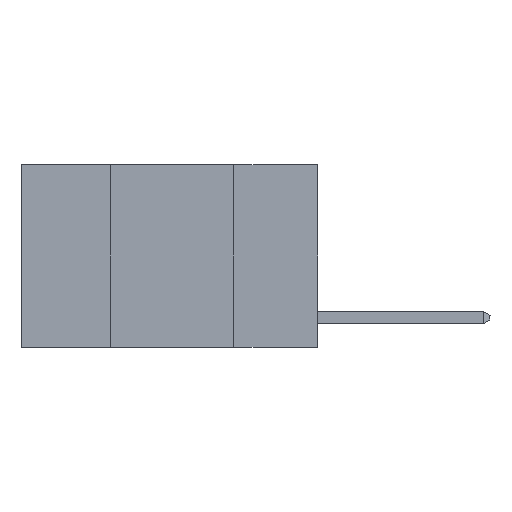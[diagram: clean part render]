
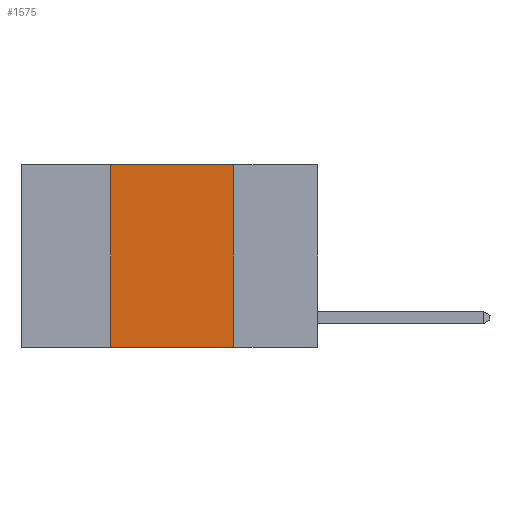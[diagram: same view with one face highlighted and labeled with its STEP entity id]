
A CAD part, left-side view. The second image highlights one B-rep face of the part: STEP entity #1575.
In plain terms, the highlighted planar face has unit normal (-1, 0, 0).
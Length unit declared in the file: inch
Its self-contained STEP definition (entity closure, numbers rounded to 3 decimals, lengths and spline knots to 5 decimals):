
#529 = VECTOR ( 'NONE', #25299, 39.37008 ) ;
#1575 = ADVANCED_FACE ( 'NONE', ( #6108 ), #21739, .F. ) ;
#1997 = LINE ( 'NONE', #19917, #529 ) ;
#3007 = VERTEX_POINT ( 'NONE', #13821 ) ;
#3085 = EDGE_CURVE ( 'NONE', #11057, #13560, #20393, .T. ) ;
#3629 = ORIENTED_EDGE ( 'NONE', *, *, #12092, .F. ) ;
#4071 = DIRECTION ( 'NONE',  ( 0., 0., -1. ) ) ;
#4110 = EDGE_LOOP ( 'NONE', ( #23858, #20177, #3629, #20662 ) ) ;
#4261 = EDGE_CURVE ( 'NONE', #12815, #3007, #12194, .T. ) ;
#6108 = FACE_OUTER_BOUND ( 'NONE', #4110, .T. ) ;
#6417 = DIRECTION ( 'NONE',  ( 0., -1., 0. ) ) ;
#6546 = CARTESIAN_POINT ( 'NONE',  ( 0., 0.6, 0. ) ) ;
#6825 = DIRECTION ( 'NONE',  ( 0., -1., 0. ) ) ;
#7036 = LINE ( 'NONE', #15425, #8098 ) ;
#8098 = VECTOR ( 'NONE', #8956, 39.37008 ) ;
#8956 = DIRECTION ( 'NONE',  ( 0., 0., 1. ) ) ;
#9853 = CARTESIAN_POINT ( 'NONE',  ( 0., 0.17, -0.37 ) ) ;
#10684 = CARTESIAN_POINT ( 'NONE',  ( 0., 0.6, -0.37 ) ) ;
#11057 = VERTEX_POINT ( 'NONE', #24647 ) ;
#11877 = CARTESIAN_POINT ( 'NONE',  ( 0., 0.6, 0. ) ) ;
#12092 = EDGE_CURVE ( 'NONE', #11057, #12815, #7036, .T. ) ;
#12194 = LINE ( 'NONE', #6546, #23670 ) ;
#12815 = VERTEX_POINT ( 'NONE', #24741 ) ;
#13560 = VERTEX_POINT ( 'NONE', #9853 ) ;
#13821 = CARTESIAN_POINT ( 'NONE',  ( 0., 0.17, 0. ) ) ;
#14023 = EDGE_CURVE ( 'NONE', #3007, #13560, #1997, .T. ) ;
#15425 = CARTESIAN_POINT ( 'NONE',  ( 0., 0.42, 0. ) ) ;
#17044 = VECTOR ( 'NONE', #6825, 39.37008 ) ;
#17867 = DIRECTION ( 'NONE',  ( 1., 0., 0. ) ) ;
#19917 = CARTESIAN_POINT ( 'NONE',  ( 0., 0.17, 0. ) ) ;
#20177 = ORIENTED_EDGE ( 'NONE', *, *, #4261, .F. ) ;
#20393 = LINE ( 'NONE', #10684, #17044 ) ;
#20662 = ORIENTED_EDGE ( 'NONE', *, *, #3085, .T. ) ;
#20708 = AXIS2_PLACEMENT_3D ( 'NONE', #11877, #17867, #4071 ) ;
#21739 = PLANE ( 'NONE',  #20708 ) ;
#23670 = VECTOR ( 'NONE', #6417, 39.37008 ) ;
#23858 = ORIENTED_EDGE ( 'NONE', *, *, #14023, .F. ) ;
#24647 = CARTESIAN_POINT ( 'NONE',  ( 0., 0.42, -0.37 ) ) ;
#24741 = CARTESIAN_POINT ( 'NONE',  ( 0., 0.42, 0. ) ) ;
#25299 = DIRECTION ( 'NONE',  ( 0., 0., -1. ) ) ;
